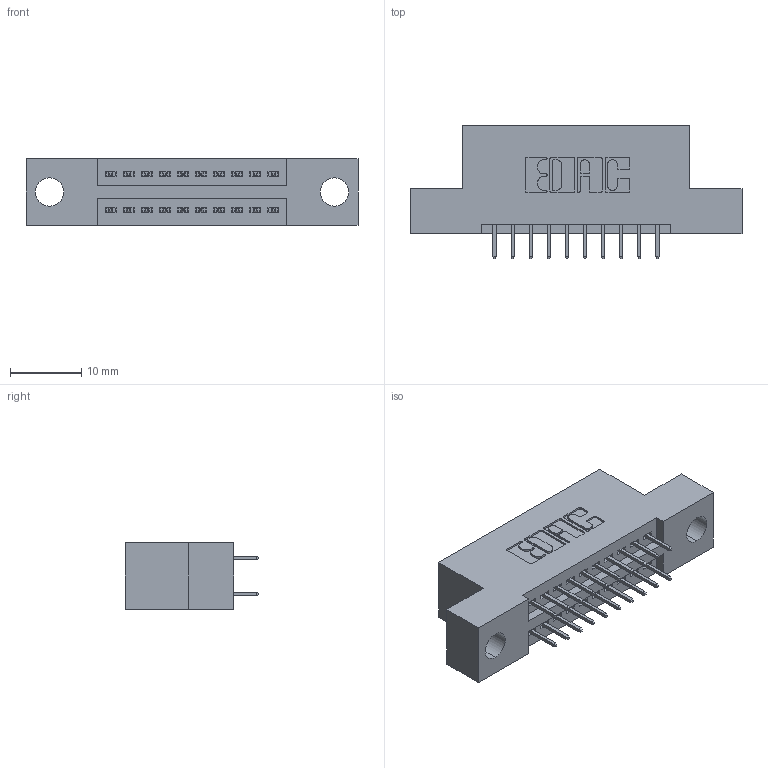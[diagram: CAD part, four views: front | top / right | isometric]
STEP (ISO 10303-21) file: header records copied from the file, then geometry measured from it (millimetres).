
FILE_DESCRIPTION (( 'STEP AP203' ), '1' );
FILE_NAME ('895-020-525-204.STEP', '2020-09-25T08:17:18', ( '' ), ( '' ), 'SwSTEP 2.0', 'SolidWorks 2020', '' );
FILE_SCHEMA (( 'CONFIG_CONTROL_DESIGN' ));
Length unit declared in the file: inch
Products named in the file (3): 895-020-525-204; 845 Part_Flush Mounting Lugs - 0.156 Dia-TH; 345-292-001_345-293-125
Assembly tree (21 placements, depth 2):
  895-020-525-204
    845 Part_Flush Mounting Lugs - 0.156 Dia-TH
    345-292-001_345-293-125  x20
Bounding box: 46.61 x 18.72 x 9.4 mm (x, y, z)
Volume: 4109.8 mm3; surface area: 5171.2 mm2
Topology: 21 solids, 21 shells, 1206 faces, 3401 edges, 2186 vertices
Faces by surface type: plane 860, cylinder 346
Entity records: 12231 total; most frequent: CARTESIAN_POINT 2080, ORIENTED_EDGE 2014, DIRECTION 1875, EDGE_CURVE 1007, VECTOR 839, LINE 839, VERTEX_POINT 666, AXIS2_PLACEMENT_3D 518
